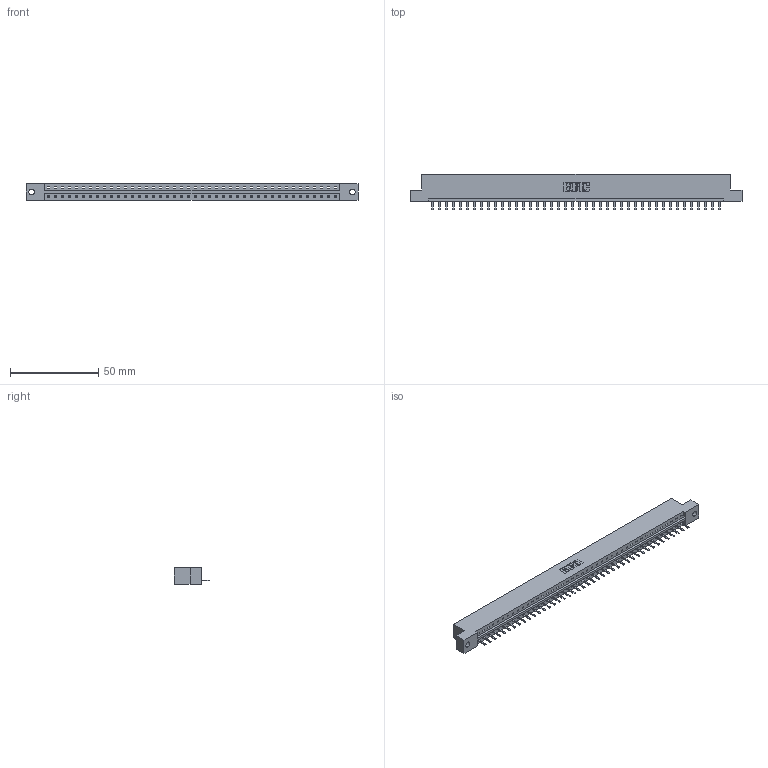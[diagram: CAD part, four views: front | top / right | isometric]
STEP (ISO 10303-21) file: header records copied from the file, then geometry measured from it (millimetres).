
FILE_DESCRIPTION (( 'STEP AP203' ), '1' );
FILE_NAME ('833-042-520-102.STEP', '2020-06-03T20:08:18', ( '' ), ( '' ), 'SwSTEP 2.0', 'SolidWorks 2020', '' );
FILE_SCHEMA (( 'CONFIG_CONTROL_DESIGN' ));
Length unit declared in the file: inch
Products named in the file (3): 833 Part_Flush - .128 Dia; 833-042-520-102; 345-292-001_345-293-120
Assembly tree (43 placements, depth 2):
  833-042-520-102
    833 Part_Flush - .128 Dia
    345-292-001_345-293-120  x42
Bounding box: 187.96 x 20.02 x 9.4 mm (x, y, z)
Volume: 18756.6 mm3; surface area: 19598.3 mm2
Topology: 43 solids, 43 shells, 2718 faces, 8039 edges, 5246 vertices
Faces by surface type: plane 1918, cylinder 800
Entity records: 25793 total; most frequent: CARTESIAN_POINT 4468, ORIENTED_EDGE 4434, DIRECTION 3757, EDGE_CURVE 2217, LINE 2085, VECTOR 2085, VERTEX_POINT 1474, AXIS2_PLACEMENT_3D 836
